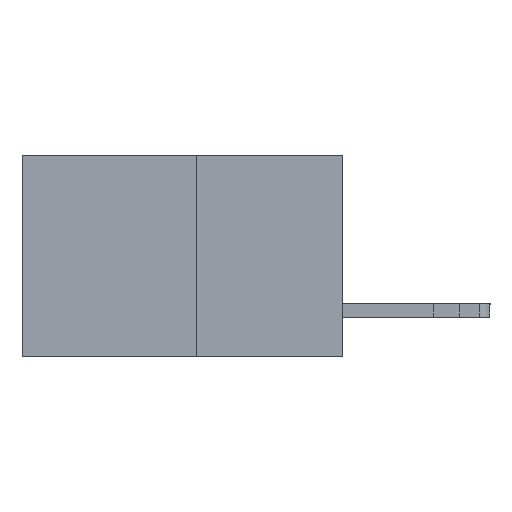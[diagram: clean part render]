
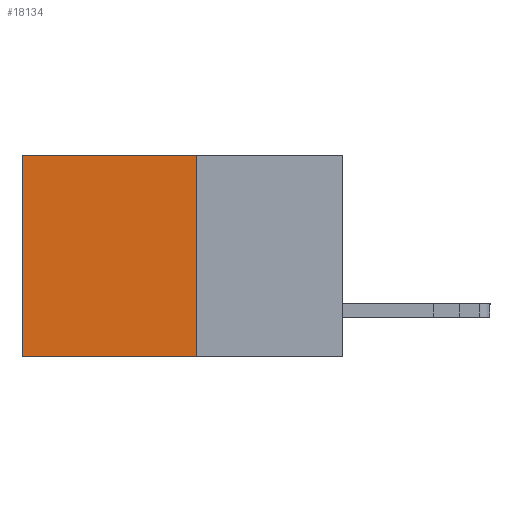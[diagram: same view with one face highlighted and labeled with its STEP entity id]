
A CAD part, left-side view. The second image highlights one B-rep face of the part: STEP entity #18134.
In plain terms, the highlighted planar face has unit normal (-1, 0, 0).
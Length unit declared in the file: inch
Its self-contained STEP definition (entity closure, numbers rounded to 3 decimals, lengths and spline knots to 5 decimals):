
#30 = CARTESIAN_POINT ( 'NONE',  ( 0.277, 0.27, -0.37 ) ) ;
#117 = DIRECTION ( 'NONE',  ( 0., 0., -1. ) ) ;
#335 = EDGE_LOOP ( 'NONE', ( #1526, #5580, #12685, #22282 ) ) ;
#1526 = ORIENTED_EDGE ( 'NONE', *, *, #20484, .T. ) ;
#2467 = DIRECTION ( 'NONE',  ( 0., 1., 0. ) ) ;
#2526 = DIRECTION ( 'NONE',  ( 0., 0., -1. ) ) ;
#3200 = EDGE_CURVE ( 'NONE', #10276, #14001, #7045, .T. ) ;
#3735 = VECTOR ( 'NONE', #2467, 39.37008 ) ;
#5580 = ORIENTED_EDGE ( 'NONE', *, *, #13621, .F. ) ;
#6648 = VERTEX_POINT ( 'NONE', #18114 ) ;
#7045 = LINE ( 'NONE', #10704, #23134 ) ;
#7213 = CARTESIAN_POINT ( 'NONE',  ( 0.277, 0.27, 0. ) ) ;
#7322 = LINE ( 'NONE', #7213, #12139 ) ;
#8998 = CARTESIAN_POINT ( 'NONE',  ( 0.277, 0.27, -0.37 ) ) ;
#9637 = CARTESIAN_POINT ( 'NONE',  ( 0.277, 0.27, 0. ) ) ;
#10276 = VERTEX_POINT ( 'NONE', #9637 ) ;
#10704 = CARTESIAN_POINT ( 'NONE',  ( 0.277, 0.27, -0.37 ) ) ;
#11174 = DIRECTION ( 'NONE',  ( 1., 0., 0. ) ) ;
#11609 = CARTESIAN_POINT ( 'NONE',  ( 0.277, 0.27, -0.37 ) ) ;
#12139 = VECTOR ( 'NONE', #21680, 39.37008 ) ;
#12685 = ORIENTED_EDGE ( 'NONE', *, *, #3200, .F. ) ;
#12992 = LINE ( 'NONE', #15274, #13556 ) ;
#13556 = VECTOR ( 'NONE', #2526, 39.37008 ) ;
#13621 = EDGE_CURVE ( 'NONE', #14001, #21642, #18259, .T. ) ;
#14001 = VERTEX_POINT ( 'NONE', #8998 ) ;
#14785 = FACE_OUTER_BOUND ( 'NONE', #335, .T. ) ;
#15274 = CARTESIAN_POINT ( 'NONE',  ( 0.277, 0.59, -0.37 ) ) ;
#17402 = CARTESIAN_POINT ( 'NONE',  ( 0.277, 0.59, -0.37 ) ) ;
#18114 = CARTESIAN_POINT ( 'NONE',  ( 0.277, 0.59, 0. ) ) ;
#18134 = ADVANCED_FACE ( 'NONE', ( #14785 ), #21945, .F. ) ;
#18259 = LINE ( 'NONE', #11609, #3735 ) ;
#20053 = DIRECTION ( 'NONE',  ( 0., 0., -1. ) ) ;
#20207 = EDGE_CURVE ( 'NONE', #10276, #6648, #7322, .T. ) ;
#20484 = EDGE_CURVE ( 'NONE', #6648, #21642, #12992, .T. ) ;
#21515 = AXIS2_PLACEMENT_3D ( 'NONE', #30, #11174, #117 ) ;
#21642 = VERTEX_POINT ( 'NONE', #17402 ) ;
#21680 = DIRECTION ( 'NONE',  ( 0., 1., 0. ) ) ;
#21945 = PLANE ( 'NONE',  #21515 ) ;
#22282 = ORIENTED_EDGE ( 'NONE', *, *, #20207, .T. ) ;
#23134 = VECTOR ( 'NONE', #20053, 39.37008 ) ;
